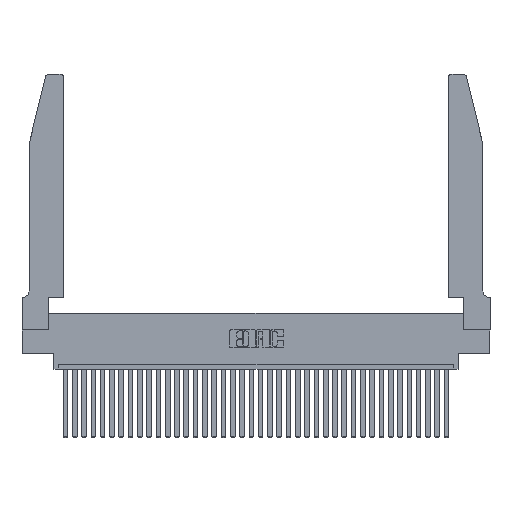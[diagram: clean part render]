
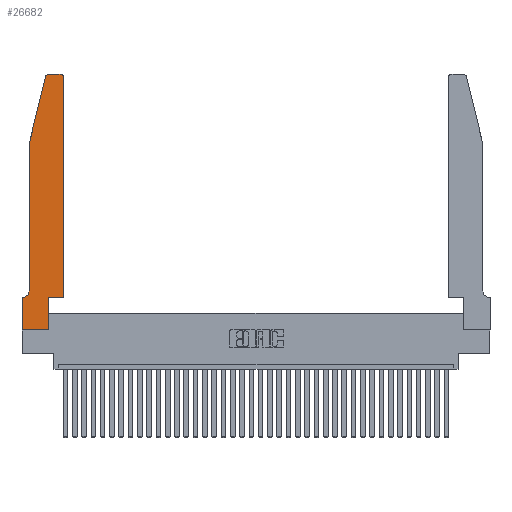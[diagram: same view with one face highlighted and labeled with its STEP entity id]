
A CAD part, top view. The second image highlights one B-rep face of the part: STEP entity #26682.
In plain terms, the highlighted planar face has unit normal (0, 0, 1).
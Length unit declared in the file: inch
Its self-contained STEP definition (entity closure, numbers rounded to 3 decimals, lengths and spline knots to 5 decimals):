
#503 = PLANE ( 'NONE',  #8943 ) ;
#836 = VERTEX_POINT ( 'NONE', #29595 ) ;
#905 = VECTOR ( 'NONE', #3465, 39.37008 ) ;
#919 = ORIENTED_EDGE ( 'NONE', *, *, #5458, .T. ) ;
#1138 = CARTESIAN_POINT ( 'NONE',  ( 0.4505, 0.35, 0.37 ) ) ;
#2390 = EDGE_CURVE ( 'NONE', #10214, #23248, #16770, .T. ) ;
#2518 = LINE ( 'NONE', #20676, #20500 ) ;
#2549 = CARTESIAN_POINT ( 'NONE',  ( 0.2865, 0., 0.37 ) ) ;
#2671 = VECTOR ( 'NONE', #20981, 39.37008 ) ;
#2875 = ORIENTED_EDGE ( 'NONE', *, *, #27343, .T. ) ;
#3346 = CARTESIAN_POINT ( 'NONE',  ( 0.0755, 0.42, 0.37 ) ) ;
#3465 = DIRECTION ( 'NONE',  ( 0., -1., 0. ) ) ;
#3711 = DIRECTION ( 'NONE',  ( 0., -1., 0. ) ) ;
#3953 = DIRECTION ( 'NONE',  ( 1., 0., 0. ) ) ;
#5458 = EDGE_CURVE ( 'NONE', #7230, #33247, #16946, .T. ) ;
#6142 = DIRECTION ( 'NONE',  ( 0., 0., 1. ) ) ;
#6593 = EDGE_CURVE ( 'NONE', #20334, #7855, #2518, .T. ) ;
#6715 = CARTESIAN_POINT ( 'NONE',  ( 0.284, 2.72, 0.37 ) ) ;
#7230 = VERTEX_POINT ( 'NONE', #16022 ) ;
#7352 = LINE ( 'NONE', #10829, #13065 ) ;
#7479 = VECTOR ( 'NONE', #3953, 39.37008 ) ;
#7575 = VECTOR ( 'NONE', #3711, 39.37008 ) ;
#7855 = VERTEX_POINT ( 'NONE', #14832 ) ;
#8528 = ORIENTED_EDGE ( 'NONE', *, *, #15202, .T. ) ;
#8548 = CARTESIAN_POINT ( 'NONE',  ( 0.284, 2.75, 0.37 ) ) ;
#8780 = CARTESIAN_POINT ( 'NONE',  ( 0.4505, 0.35, 0.37 ) ) ;
#8897 = ORIENTED_EDGE ( 'NONE', *, *, #16614, .T. ) ;
#8943 = AXIS2_PLACEMENT_3D ( 'NONE', #11802, #6142, #8987 ) ;
#8964 = VERTEX_POINT ( 'NONE', #33169 ) ;
#8987 = DIRECTION ( 'NONE',  ( 1., 0., 0. ) ) ;
#9221 = VERTEX_POINT ( 'NONE', #23070 ) ;
#9634 = EDGE_LOOP ( 'NONE', ( #919, #15133, #35386, #14202, #2875, #8897, #8528, #25923, #31298, #27978, #16253, #14691 ) ) ;
#9796 = CIRCLE ( 'NONE', #35536, 0.03 ) ;
#10214 = VERTEX_POINT ( 'NONE', #21819 ) ;
#10829 = CARTESIAN_POINT ( 'NONE',  ( 0.0755, 2., 0.37 ) ) ;
#11667 = DIRECTION ( 'NONE',  ( -0.239, -0.971, 0. ) ) ;
#11802 = CARTESIAN_POINT ( 'NONE',  ( 0., 0.35, 0.37 ) ) ;
#11890 = CARTESIAN_POINT ( 'NONE',  ( 0., 0., 0.37 ) ) ;
#12355 = DIRECTION ( 'NONE',  ( 1., 0., 0. ) ) ;
#12814 = EDGE_CURVE ( 'NONE', #836, #10214, #7352, .T. ) ;
#13065 = VECTOR ( 'NONE', #11667, 39.37008 ) ;
#13583 = CARTESIAN_POINT ( 'NONE',  ( 0.4505, 2.72, 0.37 ) ) ;
#13829 = VERTEX_POINT ( 'NONE', #13583 ) ;
#14202 = ORIENTED_EDGE ( 'NONE', *, *, #2390, .T. ) ;
#14691 = ORIENTED_EDGE ( 'NONE', *, *, #23984, .T. ) ;
#14832 = CARTESIAN_POINT ( 'NONE',  ( 0.2865, 0.35, 0.37 ) ) ;
#14862 = AXIS2_PLACEMENT_3D ( 'NONE', #25759, #17164, #32012 ) ;
#15133 = ORIENTED_EDGE ( 'NONE', *, *, #27968, .T. ) ;
#15202 = EDGE_CURVE ( 'NONE', #8964, #9221, #28160, .T. ) ;
#15526 = FACE_OUTER_BOUND ( 'NONE', #9634, .T. ) ;
#15963 = CIRCLE ( 'NONE', #20679, 0.03 ) ;
#16022 = CARTESIAN_POINT ( 'NONE',  ( 0.4205, 2.75, 0.37 ) ) ;
#16090 = DIRECTION ( 'NONE',  ( 0., 1., 0. ) ) ;
#16178 = EDGE_CURVE ( 'NONE', #9221, #20334, #28557, .T. ) ;
#16253 = ORIENTED_EDGE ( 'NONE', *, *, #35608, .T. ) ;
#16273 = VECTOR ( 'NONE', #25728, 39.37008 ) ;
#16614 = EDGE_CURVE ( 'NONE', #33233, #8964, #18436, .T. ) ;
#16770 = LINE ( 'NONE', #28375, #7575 ) ;
#16896 = CARTESIAN_POINT ( 'NONE',  ( 0.0055, 0.35, 0.37 ) ) ;
#16946 = LINE ( 'NONE', #18936, #26603 ) ;
#17164 = DIRECTION ( 'NONE',  ( 0., 0., -1. ) ) ;
#17649 = CIRCLE ( 'NONE', #14862, 0.07 ) ;
#18436 = LINE ( 'NONE', #22914, #16273 ) ;
#18936 = CARTESIAN_POINT ( 'NONE',  ( 0.2605, 2.75, 0.37 ) ) ;
#19052 = DIRECTION ( 'NONE',  ( -1., 0., 0. ) ) ;
#19634 = EDGE_CURVE ( 'NONE', #7855, #33274, #33748, .T. ) ;
#20334 = VERTEX_POINT ( 'NONE', #2549 ) ;
#20398 = LINE ( 'NONE', #21393, #29654 ) ;
#20500 = VECTOR ( 'NONE', #26073, 39.37008 ) ;
#20676 = CARTESIAN_POINT ( 'NONE',  ( 0.2865, 0.35, 0.37 ) ) ;
#20679 = AXIS2_PLACEMENT_3D ( 'NONE', #29083, #35047, #21120 ) ;
#20981 = DIRECTION ( 'NONE',  ( 1., 0., 0. ) ) ;
#21120 = DIRECTION ( 'NONE',  ( 1., 0., 0. ) ) ;
#21393 = CARTESIAN_POINT ( 'NONE',  ( 0.4505, 0.35, 0.37 ) ) ;
#21819 = CARTESIAN_POINT ( 'NONE',  ( 0.0755, 2., 0.37 ) ) ;
#22914 = CARTESIAN_POINT ( 'NONE',  ( 0.0755, 0.35, 0.37 ) ) ;
#23070 = CARTESIAN_POINT ( 'NONE',  ( 0., 0., 0.37 ) ) ;
#23248 = VERTEX_POINT ( 'NONE', #3346 ) ;
#23984 = EDGE_CURVE ( 'NONE', #13829, #7230, #15963, .T. ) ;
#25728 = DIRECTION ( 'NONE',  ( -1., 0., 0. ) ) ;
#25759 = CARTESIAN_POINT ( 'NONE',  ( 0.0055, 0.42, 0.37 ) ) ;
#25923 = ORIENTED_EDGE ( 'NONE', *, *, #16178, .T. ) ;
#26073 = DIRECTION ( 'NONE',  ( 0., 1., 0. ) ) ;
#26603 = VECTOR ( 'NONE', #19052, 39.37008 ) ;
#26682 = ADVANCED_FACE ( 'NONE', ( #15526 ), #503, .T. ) ;
#27343 = EDGE_CURVE ( 'NONE', #23248, #33233, #17649, .T. ) ;
#27968 = EDGE_CURVE ( 'NONE', #33247, #836, #9796, .T. ) ;
#27978 = ORIENTED_EDGE ( 'NONE', *, *, #19634, .T. ) ;
#28160 = LINE ( 'NONE', #30650, #905 ) ;
#28375 = CARTESIAN_POINT ( 'NONE',  ( 0.0755, 2., 0.37 ) ) ;
#28557 = LINE ( 'NONE', #11890, #2671 ) ;
#29083 = CARTESIAN_POINT ( 'NONE',  ( 0.4205, 2.72, 0.37 ) ) ;
#29172 = DIRECTION ( 'NONE',  ( 0., 0., 1. ) ) ;
#29595 = CARTESIAN_POINT ( 'NONE',  ( 0.25487, 2.72718, 0.37 ) ) ;
#29654 = VECTOR ( 'NONE', #16090, 39.37008 ) ;
#30650 = CARTESIAN_POINT ( 'NONE',  ( 0., 0., 0.37 ) ) ;
#31298 = ORIENTED_EDGE ( 'NONE', *, *, #6593, .T. ) ;
#32012 = DIRECTION ( 'NONE',  ( -1., 0., 0. ) ) ;
#33169 = CARTESIAN_POINT ( 'NONE',  ( 0., 0.35, 0.37 ) ) ;
#33233 = VERTEX_POINT ( 'NONE', #16896 ) ;
#33247 = VERTEX_POINT ( 'NONE', #8548 ) ;
#33274 = VERTEX_POINT ( 'NONE', #8780 ) ;
#33748 = LINE ( 'NONE', #1138, #7479 ) ;
#35047 = DIRECTION ( 'NONE',  ( 0., 0., 1. ) ) ;
#35386 = ORIENTED_EDGE ( 'NONE', *, *, #12814, .T. ) ;
#35536 = AXIS2_PLACEMENT_3D ( 'NONE', #6715, #29172, #12355 ) ;
#35608 = EDGE_CURVE ( 'NONE', #33274, #13829, #20398, .T. ) ;
